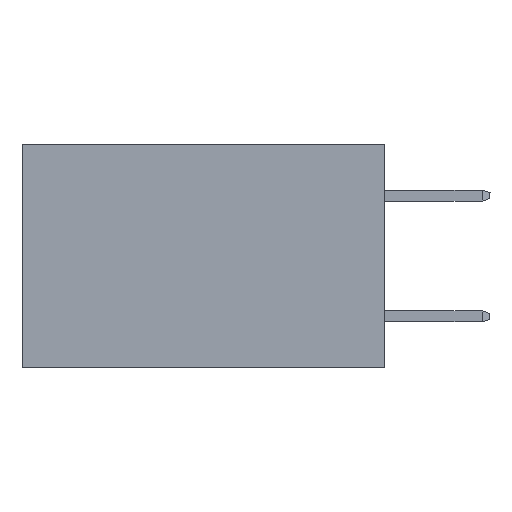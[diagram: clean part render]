
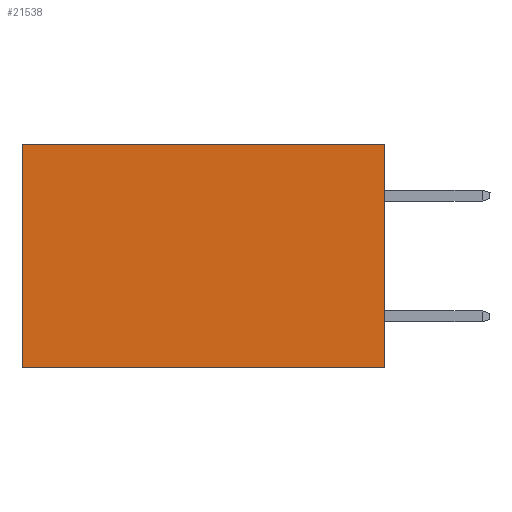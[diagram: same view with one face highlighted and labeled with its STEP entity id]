
A CAD part, left-side view. The second image highlights one B-rep face of the part: STEP entity #21538.
In plain terms, the highlighted planar face has unit normal (-1, 0, 0).
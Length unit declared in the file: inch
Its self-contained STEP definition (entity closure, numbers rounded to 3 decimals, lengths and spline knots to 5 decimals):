
#518 = EDGE_CURVE ( 'NONE', #7373, #1405, #12776, .T. ) ;
#1217 = CARTESIAN_POINT ( 'NONE',  ( 0.298, 0., 0. ) ) ;
#1405 = VERTEX_POINT ( 'NONE', #21691 ) ;
#2078 = CARTESIAN_POINT ( 'NONE',  ( 0.298, 0., 0. ) ) ;
#2368 = EDGE_CURVE ( 'NONE', #7373, #16166, #9742, .T. ) ;
#3765 = CARTESIAN_POINT ( 'NONE',  ( 0.298, 0.6, 0. ) ) ;
#5466 = VECTOR ( 'NONE', #16975, 39.37008 ) ;
#7029 = DIRECTION ( 'NONE',  ( 0., 0., -1. ) ) ;
#7373 = VERTEX_POINT ( 'NONE', #9561 ) ;
#8059 = DIRECTION ( 'NONE',  ( 0., 1., 0. ) ) ;
#8202 = CARTESIAN_POINT ( 'NONE',  ( 0.298, 0., 0. ) ) ;
#8659 = ORIENTED_EDGE ( 'NONE', *, *, #518, .F. ) ;
#9561 = CARTESIAN_POINT ( 'NONE',  ( 0.298, 0., 0. ) ) ;
#9742 = LINE ( 'NONE', #1217, #10003 ) ;
#9888 = DIRECTION ( 'NONE',  ( 0., 0., -1. ) ) ;
#10003 = VECTOR ( 'NONE', #8059, 39.37008 ) ;
#10459 = EDGE_CURVE ( 'NONE', #1405, #21861, #21859, .T. ) ;
#10902 = VECTOR ( 'NONE', #7029, 39.37008 ) ;
#11958 = DIRECTION ( 'NONE',  ( 0., 1., 0. ) ) ;
#12036 = EDGE_LOOP ( 'NONE', ( #13438, #17901, #8659, #15679 ) ) ;
#12776 = LINE ( 'NONE', #2078, #10902 ) ;
#13438 = ORIENTED_EDGE ( 'NONE', *, *, #17249, .T. ) ;
#13622 = LINE ( 'NONE', #20462, #5466 ) ;
#15201 = PLANE ( 'NONE',  #21166 ) ;
#15206 = VECTOR ( 'NONE', #11958, 39.37008 ) ;
#15679 = ORIENTED_EDGE ( 'NONE', *, *, #2368, .T. ) ;
#16166 = VERTEX_POINT ( 'NONE', #3765 ) ;
#16206 = CARTESIAN_POINT ( 'NONE',  ( 0.298, 0.6, -0.37 ) ) ;
#16975 = DIRECTION ( 'NONE',  ( 0., 0., -1. ) ) ;
#17249 = EDGE_CURVE ( 'NONE', #16166, #21861, #13622, .T. ) ;
#17901 = ORIENTED_EDGE ( 'NONE', *, *, #10459, .F. ) ;
#18976 = FACE_OUTER_BOUND ( 'NONE', #12036, .T. ) ;
#20462 = CARTESIAN_POINT ( 'NONE',  ( 0.298, 0.6, 0. ) ) ;
#21166 = AXIS2_PLACEMENT_3D ( 'NONE', #8202, #22084, #9888 ) ;
#21538 = ADVANCED_FACE ( 'NONE', ( #18976 ), #15201, .F. ) ;
#21691 = CARTESIAN_POINT ( 'NONE',  ( 0.298, 0., -0.37 ) ) ;
#21859 = LINE ( 'NONE', #22526, #15206 ) ;
#21861 = VERTEX_POINT ( 'NONE', #16206 ) ;
#22084 = DIRECTION ( 'NONE',  ( 1., 0., 0. ) ) ;
#22526 = CARTESIAN_POINT ( 'NONE',  ( 0.298, 0., -0.37 ) ) ;
